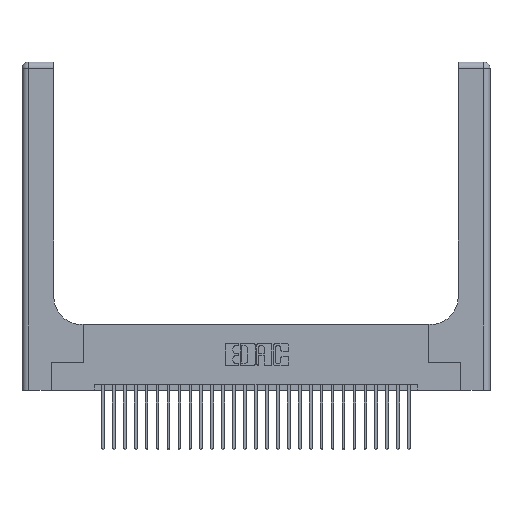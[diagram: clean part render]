
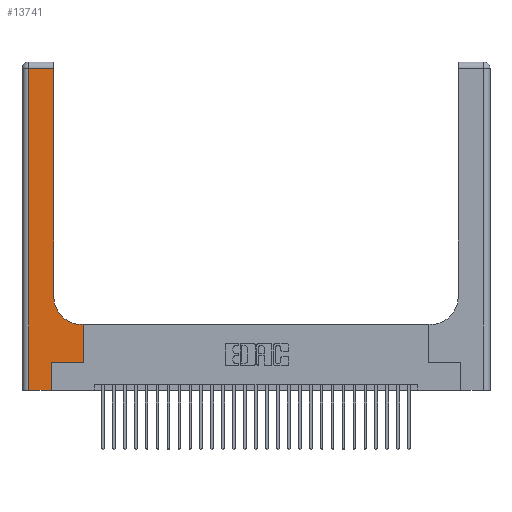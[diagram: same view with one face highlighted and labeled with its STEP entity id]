
A CAD part, top view. The second image highlights one B-rep face of the part: STEP entity #13741.
In plain terms, the highlighted planar face has unit normal (0, 0, 1).
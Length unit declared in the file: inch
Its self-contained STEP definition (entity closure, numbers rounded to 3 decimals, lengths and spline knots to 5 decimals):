
#1164 = ORIENTED_EDGE ( 'NONE', *, *, #3113, .T. ) ;
#1247 = CARTESIAN_POINT ( 'NONE',  ( 0.5585, 0.25, 0.37 ) ) ;
#1400 = DIRECTION ( 'NONE',  ( 1., 0., 0. ) ) ;
#1748 = LINE ( 'NONE', #27275, #25435 ) ;
#2053 = EDGE_CURVE ( 'NONE', #7773, #3117, #13869, .T. ) ;
#2372 = VERTEX_POINT ( 'NONE', #25407 ) ;
#2590 = CARTESIAN_POINT ( 'NONE',  ( 0.06, 0., 0.37 ) ) ;
#3113 = EDGE_CURVE ( 'NONE', #2372, #7773, #21574, .T. ) ;
#3117 = VERTEX_POINT ( 'NONE', #28484 ) ;
#4414 = VERTEX_POINT ( 'NONE', #13019 ) ;
#4489 = CARTESIAN_POINT ( 'NONE',  ( 0.5415, 0.6, 0.37 ) ) ;
#4664 = DIRECTION ( 'NONE',  ( -1., 0., 0. ) ) ;
#4680 = ORIENTED_EDGE ( 'NONE', *, *, #14989, .T. ) ;
#4695 = CIRCLE ( 'NONE', #27730, 0.25 ) ;
#5397 = VERTEX_POINT ( 'NONE', #20725 ) ;
#6719 = VERTEX_POINT ( 'NONE', #12464 ) ;
#7105 = VECTOR ( 'NONE', #12438, 39.37008 ) ;
#7233 = CARTESIAN_POINT ( 'NONE',  ( 0.2915, 2.94, 0.37 ) ) ;
#7373 = DIRECTION ( 'NONE',  ( 0., 1., 0. ) ) ;
#7666 = VECTOR ( 'NONE', #24441, 39.37008 ) ;
#7773 = VERTEX_POINT ( 'NONE', #2590 ) ;
#8524 = CARTESIAN_POINT ( 'NONE',  ( 0., 0., 0.37 ) ) ;
#8574 = LINE ( 'NONE', #16986, #7105 ) ;
#8955 = VERTEX_POINT ( 'NONE', #7233 ) ;
#9141 = VECTOR ( 'NONE', #7373, 39.37008 ) ;
#9283 = VERTEX_POINT ( 'NONE', #1247 ) ;
#9449 = ORIENTED_EDGE ( 'NONE', *, *, #14108, .T. ) ;
#9896 = CARTESIAN_POINT ( 'NONE',  ( 0., 3., 0.37 ) ) ;
#10335 = CARTESIAN_POINT ( 'NONE',  ( 0.06, 3., 0.37 ) ) ;
#11277 = ORIENTED_EDGE ( 'NONE', *, *, #16156, .T. ) ;
#11314 = ORIENTED_EDGE ( 'NONE', *, *, #26427, .T. ) ;
#11709 = CARTESIAN_POINT ( 'NONE',  ( 0., 2.94, 0.37 ) ) ;
#11758 = CARTESIAN_POINT ( 'NONE',  ( 0.2915, 0.6, 0.37 ) ) ;
#12220 = DIRECTION ( 'NONE',  ( 0., 0., -1. ) ) ;
#12438 = DIRECTION ( 'NONE',  ( 0., 1., 0. ) ) ;
#12464 = CARTESIAN_POINT ( 'NONE',  ( 0.269, 0.25, 0.37 ) ) ;
#12634 = DIRECTION ( 'NONE',  ( -1., 0., 0. ) ) ;
#12949 = VECTOR ( 'NONE', #1400, 39.37008 ) ;
#13019 = CARTESIAN_POINT ( 'NONE',  ( 0.5585, 0.6, 0.37 ) ) ;
#13062 = CARTESIAN_POINT ( 'NONE',  ( 0.269, 0.25, 0.37 ) ) ;
#13741 = ADVANCED_FACE ( 'NONE', ( #22188 ), #21663, .F. ) ;
#13869 = LINE ( 'NONE', #8524, #7666 ) ;
#14108 = EDGE_CURVE ( 'NONE', #6719, #9283, #24956, .T. ) ;
#14575 = LINE ( 'NONE', #21109, #9141 ) ;
#14989 = EDGE_CURVE ( 'NONE', #8955, #2372, #27038, .T. ) ;
#16011 = AXIS2_PLACEMENT_3D ( 'NONE', #9896, #26141, #12634 ) ;
#16088 = ORIENTED_EDGE ( 'NONE', *, *, #18731, .T. ) ;
#16156 = EDGE_CURVE ( 'NONE', #4414, #17865, #23453, .T. ) ;
#16304 = DIRECTION ( 'NONE',  ( -1., 0., 0. ) ) ;
#16986 = CARTESIAN_POINT ( 'NONE',  ( 0.2915, 3., 0.37 ) ) ;
#17861 = EDGE_CURVE ( 'NONE', #3117, #6719, #1748, .T. ) ;
#17865 = VERTEX_POINT ( 'NONE', #4489 ) ;
#18731 = EDGE_CURVE ( 'NONE', #17865, #5397, #4695, .T. ) ;
#19291 = ORIENTED_EDGE ( 'NONE', *, *, #24406, .T. ) ;
#20725 = CARTESIAN_POINT ( 'NONE',  ( 0.2915, 0.85, 0.37 ) ) ;
#21109 = CARTESIAN_POINT ( 'NONE',  ( 0.5585, 0.25, 0.37 ) ) ;
#21574 = LINE ( 'NONE', #10335, #22264 ) ;
#21663 = PLANE ( 'NONE',  #16011 ) ;
#22188 = FACE_OUTER_BOUND ( 'NONE', #27026, .T. ) ;
#22264 = VECTOR ( 'NONE', #26178, 39.37008 ) ;
#23453 = LINE ( 'NONE', #11758, #26587 ) ;
#24406 = EDGE_CURVE ( 'NONE', #9283, #4414, #14575, .T. ) ;
#24441 = DIRECTION ( 'NONE',  ( 1., 0., 0. ) ) ;
#24956 = LINE ( 'NONE', #13062, #12949 ) ;
#24993 = DIRECTION ( 'NONE',  ( 0., 1., 0. ) ) ;
#25407 = CARTESIAN_POINT ( 'NONE',  ( 0.06, 2.94, 0.37 ) ) ;
#25435 = VECTOR ( 'NONE', #24993, 39.37008 ) ;
#25734 = CARTESIAN_POINT ( 'NONE',  ( 0.5415, 0.85, 0.37 ) ) ;
#26141 = DIRECTION ( 'NONE',  ( 0., 0., -1. ) ) ;
#26178 = DIRECTION ( 'NONE',  ( 0., -1., 0. ) ) ;
#26301 = VECTOR ( 'NONE', #4664, 39.37008 ) ;
#26427 = EDGE_CURVE ( 'NONE', #5397, #8955, #8574, .T. ) ;
#26587 = VECTOR ( 'NONE', #16304, 39.37008 ) ;
#27026 = EDGE_LOOP ( 'NONE', ( #11314, #4680, #1164, #29622, #27746, #9449, #19291, #11277, #16088 ) ) ;
#27038 = LINE ( 'NONE', #11709, #26301 ) ;
#27275 = CARTESIAN_POINT ( 'NONE',  ( 0.269, 0., 0.37 ) ) ;
#27730 = AXIS2_PLACEMENT_3D ( 'NONE', #25734, #12220, #28017 ) ;
#27746 = ORIENTED_EDGE ( 'NONE', *, *, #17861, .T. ) ;
#28017 = DIRECTION ( 'NONE',  ( 1., 0., 0. ) ) ;
#28484 = CARTESIAN_POINT ( 'NONE',  ( 0.269, 0., 0.37 ) ) ;
#29622 = ORIENTED_EDGE ( 'NONE', *, *, #2053, .T. ) ;
